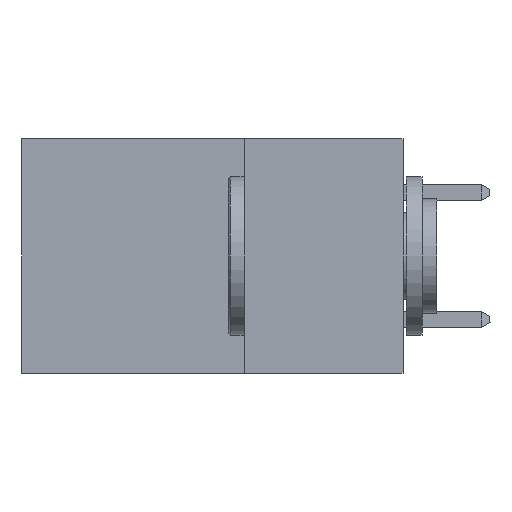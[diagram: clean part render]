
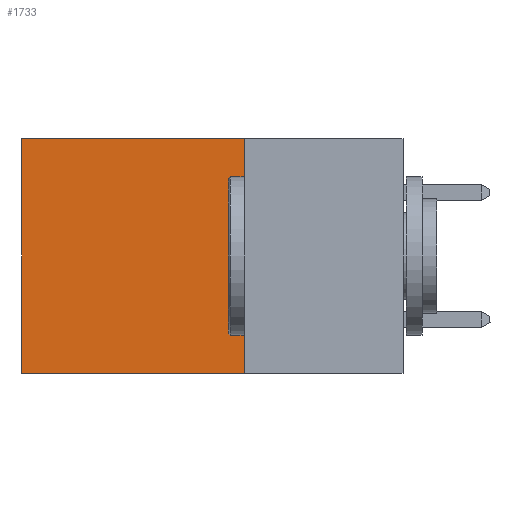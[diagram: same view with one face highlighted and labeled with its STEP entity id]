
A CAD part, left-side view. The second image highlights one B-rep face of the part: STEP entity #1733.
In plain terms, the highlighted planar face has unit normal (-1, 0, 0).
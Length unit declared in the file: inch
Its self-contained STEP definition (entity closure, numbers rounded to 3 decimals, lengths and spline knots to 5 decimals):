
#1116 = LINE ( 'NONE', #10315, #10478 ) ;
#1557 = DIRECTION ( 'NONE',  ( 0., 0., -1. ) ) ;
#1733 = ADVANCED_FACE ( 'NONE', ( #14116 ), #21141, .F. ) ;
#2344 = ORIENTED_EDGE ( 'NONE', *, *, #9317, .F. ) ;
#3821 = CARTESIAN_POINT ( 'NONE',  ( 0.2875, 0.6, -0.37 ) ) ;
#3925 = LINE ( 'NONE', #5225, #13649 ) ;
#4145 = CARTESIAN_POINT ( 'NONE',  ( 0.2875, 0.25, 0. ) ) ;
#5225 = CARTESIAN_POINT ( 'NONE',  ( 0.2875, 0.25, 0. ) ) ;
#5509 = CARTESIAN_POINT ( 'NONE',  ( 0.2875, 0.25, -0.37 ) ) ;
#5800 = VECTOR ( 'NONE', #8250, 39.37008 ) ;
#5921 = LINE ( 'NONE', #5509, #15935 ) ;
#7573 = CARTESIAN_POINT ( 'NONE',  ( 0.2875, 0.25, -0.37 ) ) ;
#8250 = DIRECTION ( 'NONE',  ( 0., 0., -1. ) ) ;
#8692 = AXIS2_PLACEMENT_3D ( 'NONE', #17330, #9359, #1557 ) ;
#9317 = EDGE_CURVE ( 'NONE', #18924, #17767, #1116, .T. ) ;
#9359 = DIRECTION ( 'NONE',  ( 1., 0., 0. ) ) ;
#10315 = CARTESIAN_POINT ( 'NONE',  ( 0.2875, 0.25, 0. ) ) ;
#10478 = VECTOR ( 'NONE', #20150, 39.37008 ) ;
#11983 = ORIENTED_EDGE ( 'NONE', *, *, #19544, .T. ) ;
#12228 = CARTESIAN_POINT ( 'NONE',  ( 0.2875, 0.6, 0. ) ) ;
#13555 = ORIENTED_EDGE ( 'NONE', *, *, #20203, .T. ) ;
#13649 = VECTOR ( 'NONE', #22841, 39.37008 ) ;
#14116 = FACE_OUTER_BOUND ( 'NONE', #17245, .T. ) ;
#15935 = VECTOR ( 'NONE', #23660, 39.37008 ) ;
#16756 = EDGE_CURVE ( 'NONE', #17767, #22397, #5921, .T. ) ;
#16795 = LINE ( 'NONE', #12228, #5800 ) ;
#17245 = EDGE_LOOP ( 'NONE', ( #13555, #20492, #2344, #11983 ) ) ;
#17330 = CARTESIAN_POINT ( 'NONE',  ( 0.2875, 0.25, 0. ) ) ;
#17767 = VERTEX_POINT ( 'NONE', #7573 ) ;
#18390 = VERTEX_POINT ( 'NONE', #20480 ) ;
#18924 = VERTEX_POINT ( 'NONE', #4145 ) ;
#19544 = EDGE_CURVE ( 'NONE', #18924, #18390, #3925, .T. ) ;
#20150 = DIRECTION ( 'NONE',  ( 0., 0., -1. ) ) ;
#20203 = EDGE_CURVE ( 'NONE', #18390, #22397, #16795, .T. ) ;
#20480 = CARTESIAN_POINT ( 'NONE',  ( 0.2875, 0.6, 0. ) ) ;
#20492 = ORIENTED_EDGE ( 'NONE', *, *, #16756, .F. ) ;
#21141 = PLANE ( 'NONE',  #8692 ) ;
#22397 = VERTEX_POINT ( 'NONE', #3821 ) ;
#22841 = DIRECTION ( 'NONE',  ( 0., 1., 0. ) ) ;
#23660 = DIRECTION ( 'NONE',  ( 0., 1., 0. ) ) ;
